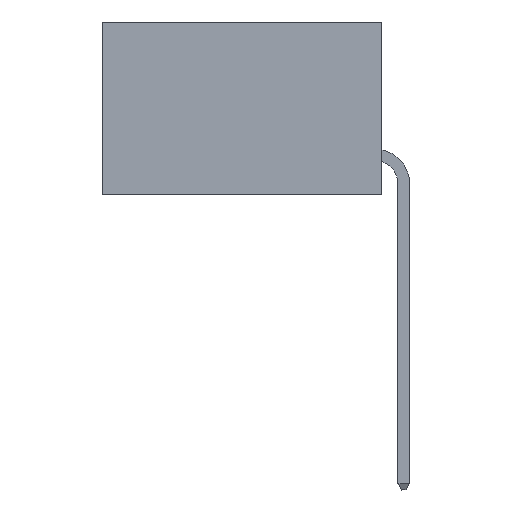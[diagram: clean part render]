
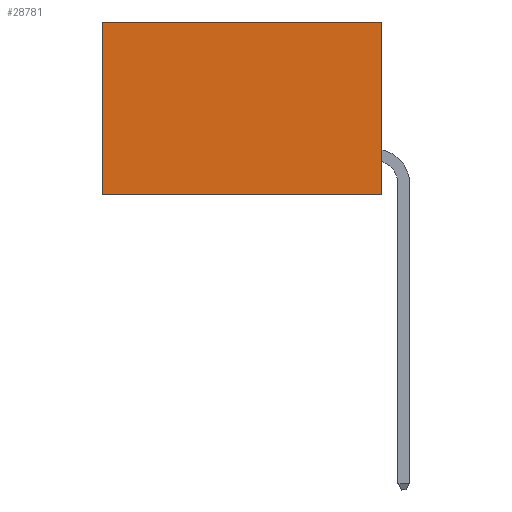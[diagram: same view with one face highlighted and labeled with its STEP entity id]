
A CAD part, left-side view. The second image highlights one B-rep face of the part: STEP entity #28781.
In plain terms, the highlighted planar face has unit normal (-1, 0, 0).
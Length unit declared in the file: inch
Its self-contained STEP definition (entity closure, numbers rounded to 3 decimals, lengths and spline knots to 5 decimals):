
#2001 = CARTESIAN_POINT ( 'NONE',  ( 0.2875, 0., 0. ) ) ;
#2145 = ORIENTED_EDGE ( 'NONE', *, *, #5589, .F. ) ;
#3795 = VERTEX_POINT ( 'NONE', #31711 ) ;
#3936 = ORIENTED_EDGE ( 'NONE', *, *, #30640, .T. ) ;
#4009 = DIRECTION ( 'NONE',  ( 0., 1., 0. ) ) ;
#4195 = VECTOR ( 'NONE', #4009, 39.37008 ) ;
#4999 = CARTESIAN_POINT ( 'NONE',  ( 0.2875, 0.6, 0. ) ) ;
#5169 = ORIENTED_EDGE ( 'NONE', *, *, #22689, .T. ) ;
#5589 = EDGE_CURVE ( 'NONE', #7395, #16767, #13793, .T. ) ;
#7146 = ORIENTED_EDGE ( 'NONE', *, *, #24369, .F. ) ;
#7395 = VERTEX_POINT ( 'NONE', #13728 ) ;
#8453 = DIRECTION ( 'NONE',  ( 1., 0., 0. ) ) ;
#9626 = VECTOR ( 'NONE', #34881, 39.37008 ) ;
#10379 = LINE ( 'NONE', #19569, #27251 ) ;
#13728 = CARTESIAN_POINT ( 'NONE',  ( 0.2875, 0., -0.37 ) ) ;
#13793 = LINE ( 'NONE', #29573, #4195 ) ;
#14221 = LINE ( 'NONE', #4999, #26942 ) ;
#16767 = VERTEX_POINT ( 'NONE', #35511 ) ;
#19195 = LINE ( 'NONE', #32091, #9626 ) ;
#19305 = FACE_OUTER_BOUND ( 'NONE', #34745, .T. ) ;
#19379 = VERTEX_POINT ( 'NONE', #2001 ) ;
#19569 = CARTESIAN_POINT ( 'NONE',  ( 0.2875, 0., 0. ) ) ;
#19897 = PLANE ( 'NONE',  #22987 ) ;
#19940 = DIRECTION ( 'NONE',  ( 0., 0., -1. ) ) ;
#22689 = EDGE_CURVE ( 'NONE', #19379, #3795, #19195, .T. ) ;
#22987 = AXIS2_PLACEMENT_3D ( 'NONE', #31816, #8453, #25750 ) ;
#24369 = EDGE_CURVE ( 'NONE', #19379, #7395, #10379, .T. ) ;
#25114 = DIRECTION ( 'NONE',  ( 0., 0., -1. ) ) ;
#25750 = DIRECTION ( 'NONE',  ( 0., 0., -1. ) ) ;
#26942 = VECTOR ( 'NONE', #25114, 39.37008 ) ;
#27251 = VECTOR ( 'NONE', #19940, 39.37008 ) ;
#28781 = ADVANCED_FACE ( 'NONE', ( #19305 ), #19897, .F. ) ;
#29573 = CARTESIAN_POINT ( 'NONE',  ( 0.2875, 0., -0.37 ) ) ;
#30640 = EDGE_CURVE ( 'NONE', #3795, #16767, #14221, .T. ) ;
#31711 = CARTESIAN_POINT ( 'NONE',  ( 0.2875, 0.6, 0. ) ) ;
#31816 = CARTESIAN_POINT ( 'NONE',  ( 0.2875, 0., 0. ) ) ;
#32091 = CARTESIAN_POINT ( 'NONE',  ( 0.2875, 0., 0. ) ) ;
#34745 = EDGE_LOOP ( 'NONE', ( #3936, #2145, #7146, #5169 ) ) ;
#34881 = DIRECTION ( 'NONE',  ( 0., 1., 0. ) ) ;
#35511 = CARTESIAN_POINT ( 'NONE',  ( 0.2875, 0.6, -0.37 ) ) ;
